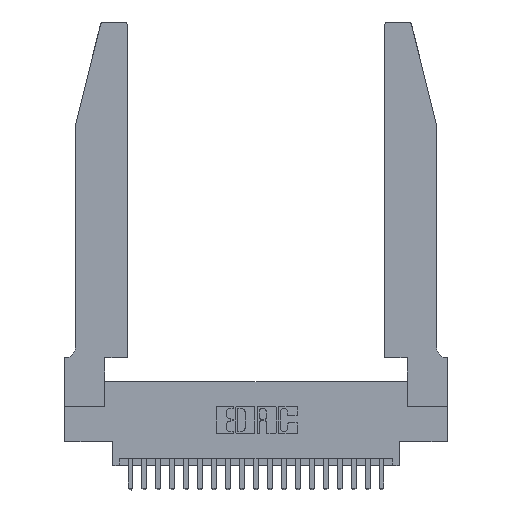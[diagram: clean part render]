
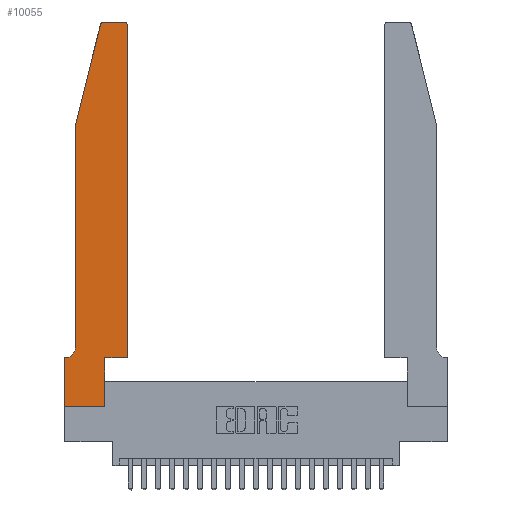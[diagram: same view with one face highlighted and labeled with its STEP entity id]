
A CAD part, top view. The second image highlights one B-rep face of the part: STEP entity #10055.
In plain terms, the highlighted planar face has unit normal (0, 0, 1).
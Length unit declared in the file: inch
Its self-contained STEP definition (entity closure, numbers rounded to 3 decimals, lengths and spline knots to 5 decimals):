
#282 = VERTEX_POINT ( 'NONE', #21796 ) ;
#558 = DIRECTION ( 'NONE',  ( 0., 0., 1. ) ) ;
#571 = DIRECTION ( 'NONE',  ( 0., 0., -1. ) ) ;
#751 = EDGE_CURVE ( 'NONE', #9058, #282, #9738, .T. ) ;
#1514 = VERTEX_POINT ( 'NONE', #20938 ) ;
#1703 = ORIENTED_EDGE ( 'NONE', *, *, #6748, .T. ) ;
#1887 = VERTEX_POINT ( 'NONE', #16844 ) ;
#2166 = CARTESIAN_POINT ( 'NONE',  ( 0.4205, 2.72, 0.37 ) ) ;
#2170 = VERTEX_POINT ( 'NONE', #18081 ) ;
#2216 = EDGE_CURVE ( 'NONE', #1887, #20005, #12536, .T. ) ;
#2514 = DIRECTION ( 'NONE',  ( -1., 0., 0. ) ) ;
#2699 = VECTOR ( 'NONE', #15063, 39.37008 ) ;
#3164 = DIRECTION ( 'NONE',  ( 0., 0., 1. ) ) ;
#3298 = AXIS2_PLACEMENT_3D ( 'NONE', #18207, #558, #20013 ) ;
#3382 = CARTESIAN_POINT ( 'NONE',  ( 0.284, 2.72, 0.37 ) ) ;
#3532 = VERTEX_POINT ( 'NONE', #16603 ) ;
#3543 = CARTESIAN_POINT ( 'NONE',  ( 0.0755, 2., 0.37 ) ) ;
#3608 = ORIENTED_EDGE ( 'NONE', *, *, #13580, .T. ) ;
#3648 = VERTEX_POINT ( 'NONE', #6860 ) ;
#3929 = ORIENTED_EDGE ( 'NONE', *, *, #5504, .T. ) ;
#4253 = EDGE_CURVE ( 'NONE', #21500, #9058, #19682, .T. ) ;
#4354 = LINE ( 'NONE', #3543, #21049 ) ;
#4427 = LINE ( 'NONE', #9745, #17492 ) ;
#4948 = LINE ( 'NONE', #16879, #16382 ) ;
#5504 = EDGE_CURVE ( 'NONE', #282, #14815, #18556, .T. ) ;
#5824 = ORIENTED_EDGE ( 'NONE', *, *, #6783, .T. ) ;
#5863 = VECTOR ( 'NONE', #12953, 39.37008 ) ;
#5980 = EDGE_CURVE ( 'NONE', #22400, #1887, #4354, .T. ) ;
#6748 = EDGE_CURVE ( 'NONE', #3532, #22400, #14560, .T. ) ;
#6783 = EDGE_CURVE ( 'NONE', #14815, #1514, #8775, .T. ) ;
#6860 = CARTESIAN_POINT ( 'NONE',  ( 0., 0.35, 0.37 ) ) ;
#7134 = EDGE_CURVE ( 'NONE', #10620, #21500, #15686, .T. ) ;
#7653 = DIRECTION ( 'NONE',  ( -1., 0., 0. ) ) ;
#7774 = EDGE_LOOP ( 'NONE', ( #20481, #17411, #1703, #14297, #13240, #21265, #3608, #21437, #23031, #12774, #3929, #5824 ) ) ;
#8278 = CARTESIAN_POINT ( 'NONE',  ( 0.0055, 0.35, 0.37 ) ) ;
#8775 = CIRCLE ( 'NONE', #17246, 0.03 ) ;
#9058 = VERTEX_POINT ( 'NONE', #19914 ) ;
#9320 = VECTOR ( 'NONE', #21525, 39.37008 ) ;
#9493 = CARTESIAN_POINT ( 'NONE',  ( 0.4505, 0.35, 0.37 ) ) ;
#9512 = CARTESIAN_POINT ( 'NONE',  ( 0.4505, 0.35, 0.37 ) ) ;
#9705 = VECTOR ( 'NONE', #20547, 39.37008 ) ;
#9738 = LINE ( 'NONE', #9493, #18045 ) ;
#9745 = CARTESIAN_POINT ( 'NONE',  ( 0.2605, 2.75, 0.37 ) ) ;
#10055 = ADVANCED_FACE ( 'NONE', ( #12414 ), #18530, .T. ) ;
#10620 = VERTEX_POINT ( 'NONE', #14804 ) ;
#10748 = CARTESIAN_POINT ( 'NONE',  ( 0.0755, 2., 0.37 ) ) ;
#10909 = CIRCLE ( 'NONE', #19026, 0.03 ) ;
#10995 = VECTOR ( 'NONE', #19112, 39.37008 ) ;
#11370 = DIRECTION ( 'NONE',  ( 1., 0., 0. ) ) ;
#12036 = LINE ( 'NONE', #22067, #5863 ) ;
#12414 = FACE_OUTER_BOUND ( 'NONE', #7774, .T. ) ;
#12536 = CIRCLE ( 'NONE', #18814, 0.07 ) ;
#12774 = ORIENTED_EDGE ( 'NONE', *, *, #751, .T. ) ;
#12953 = DIRECTION ( 'NONE',  ( 0., -1., 0. ) ) ;
#13240 = ORIENTED_EDGE ( 'NONE', *, *, #2216, .T. ) ;
#13580 = EDGE_CURVE ( 'NONE', #3648, #10620, #12036, .T. ) ;
#13992 = DIRECTION ( 'NONE',  ( 1., 0., 0. ) ) ;
#14297 = ORIENTED_EDGE ( 'NONE', *, *, #5980, .T. ) ;
#14341 = DIRECTION ( 'NONE',  ( 0., 0., 1. ) ) ;
#14560 = LINE ( 'NONE', #10748, #9320 ) ;
#14564 = DIRECTION ( 'NONE',  ( 1., 0., 0. ) ) ;
#14568 = CARTESIAN_POINT ( 'NONE',  ( 0.4505, 2.72, 0.37 ) ) ;
#14804 = CARTESIAN_POINT ( 'NONE',  ( 0., 0., 0.37 ) ) ;
#14815 = VERTEX_POINT ( 'NONE', #14568 ) ;
#15063 = DIRECTION ( 'NONE',  ( 0., 1., 0. ) ) ;
#15406 = EDGE_CURVE ( 'NONE', #20005, #3648, #4948, .T. ) ;
#15686 = LINE ( 'NONE', #20910, #10995 ) ;
#16382 = VECTOR ( 'NONE', #2514, 39.37008 ) ;
#16603 = CARTESIAN_POINT ( 'NONE',  ( 0.25487, 2.72718, 0.37 ) ) ;
#16673 = CARTESIAN_POINT ( 'NONE',  ( 0.0055, 0.42, 0.37 ) ) ;
#16844 = CARTESIAN_POINT ( 'NONE',  ( 0.0755, 0.42, 0.37 ) ) ;
#16879 = CARTESIAN_POINT ( 'NONE',  ( 0.0755, 0.35, 0.37 ) ) ;
#17246 = AXIS2_PLACEMENT_3D ( 'NONE', #2166, #14341, #14564 ) ;
#17411 = ORIENTED_EDGE ( 'NONE', *, *, #17678, .T. ) ;
#17492 = VECTOR ( 'NONE', #22306, 39.37008 ) ;
#17678 = EDGE_CURVE ( 'NONE', #2170, #3532, #10909, .T. ) ;
#18045 = VECTOR ( 'NONE', #11370, 39.37008 ) ;
#18081 = CARTESIAN_POINT ( 'NONE',  ( 0.284, 2.75, 0.37 ) ) ;
#18207 = CARTESIAN_POINT ( 'NONE',  ( 0., 0.35, 0.37 ) ) ;
#18530 = PLANE ( 'NONE',  #3298 ) ;
#18556 = LINE ( 'NONE', #9512, #2699 ) ;
#18678 = EDGE_CURVE ( 'NONE', #1514, #2170, #4427, .T. ) ;
#18814 = AXIS2_PLACEMENT_3D ( 'NONE', #16673, #571, #7653 ) ;
#19026 = AXIS2_PLACEMENT_3D ( 'NONE', #3382, #3164, #13992 ) ;
#19112 = DIRECTION ( 'NONE',  ( 1., 0., 0. ) ) ;
#19682 = LINE ( 'NONE', #19737, #9705 ) ;
#19737 = CARTESIAN_POINT ( 'NONE',  ( 0.2865, 0.35, 0.37 ) ) ;
#19914 = CARTESIAN_POINT ( 'NONE',  ( 0.2865, 0.35, 0.37 ) ) ;
#20005 = VERTEX_POINT ( 'NONE', #8278 ) ;
#20013 = DIRECTION ( 'NONE',  ( 1., 0., 0. ) ) ;
#20323 = CARTESIAN_POINT ( 'NONE',  ( 0.2865, 0., 0.37 ) ) ;
#20481 = ORIENTED_EDGE ( 'NONE', *, *, #18678, .T. ) ;
#20547 = DIRECTION ( 'NONE',  ( 0., 1., 0. ) ) ;
#20910 = CARTESIAN_POINT ( 'NONE',  ( 0., 0., 0.37 ) ) ;
#20938 = CARTESIAN_POINT ( 'NONE',  ( 0.4205, 2.75, 0.37 ) ) ;
#21049 = VECTOR ( 'NONE', #22877, 39.37008 ) ;
#21265 = ORIENTED_EDGE ( 'NONE', *, *, #15406, .T. ) ;
#21437 = ORIENTED_EDGE ( 'NONE', *, *, #7134, .T. ) ;
#21500 = VERTEX_POINT ( 'NONE', #20323 ) ;
#21525 = DIRECTION ( 'NONE',  ( -0.239, -0.971, 0. ) ) ;
#21796 = CARTESIAN_POINT ( 'NONE',  ( 0.4505, 0.35, 0.37 ) ) ;
#22067 = CARTESIAN_POINT ( 'NONE',  ( 0., 0., 0.37 ) ) ;
#22107 = CARTESIAN_POINT ( 'NONE',  ( 0.0755, 2., 0.37 ) ) ;
#22306 = DIRECTION ( 'NONE',  ( -1., 0., 0. ) ) ;
#22400 = VERTEX_POINT ( 'NONE', #22107 ) ;
#22877 = DIRECTION ( 'NONE',  ( 0., -1., 0. ) ) ;
#23031 = ORIENTED_EDGE ( 'NONE', *, *, #4253, .T. ) ;
